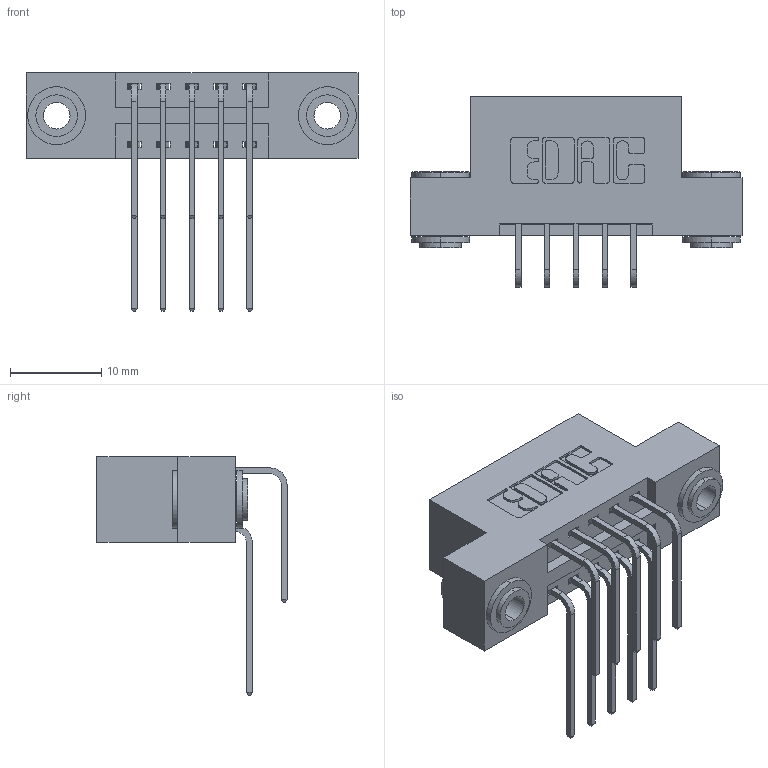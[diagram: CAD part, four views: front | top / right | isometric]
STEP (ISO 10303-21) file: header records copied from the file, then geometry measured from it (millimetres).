
FILE_DESCRIPTION (( 'STEP AP203' ), '1' );
FILE_NAME ('346-010-559-203.STEP', '2018-08-17T08:02:41', ( '' ), ( '' ), 'SwSTEP 2.0', 'SolidWorks 2016', '' );
FILE_SCHEMA (( 'CONFIG_CONTROL_DESIGN' ));
Length unit declared in the file: inch
Products named in the file (5): 346-010-559-203; 346 Part_Flush Mounting Lugs - 0.156 Dia-TH; 345-292-001_558 559 Tail - 1; 345-292-001_559 Tail - 2; 345-250-002_345-250-002-102
Assembly tree (13 placements, depth 2):
  346-010-559-203
    346 Part_Flush Mounting Lugs - 0.156 Dia-TH
    345-292-001_558 559 Tail - 1  x5
    345-292-001_559 Tail - 2  x5
    345-250-002_345-250-002-102  x2
Bounding box: 36.45 x 20.89 x 26.16 mm (x, y, z)
Volume: 3343.9 mm3; surface area: 4505.8 mm2
Topology: 13 solids, 13 shells, 700 faces, 2015 edges, 1326 vertices
Faces by surface type: plane 456, cylinder 236, cone 8
Entity records: 10678 total; most frequent: CARTESIAN_POINT 1838, ORIENTED_EDGE 1714, DIRECTION 1675, EDGE_CURVE 857, VECTOR 641, LINE 641, VERTEX_POINT 566, AXIS2_PLACEMENT_3D 517
